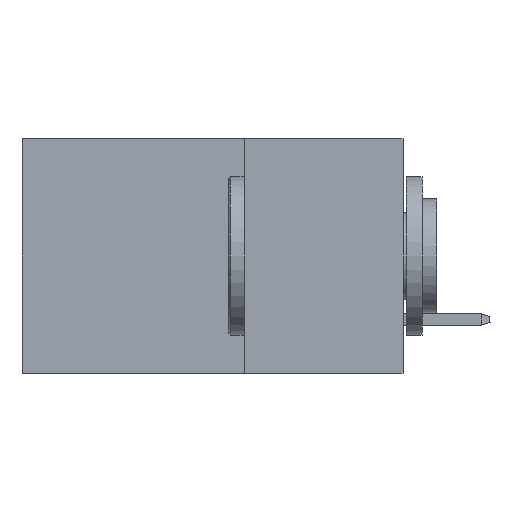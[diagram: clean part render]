
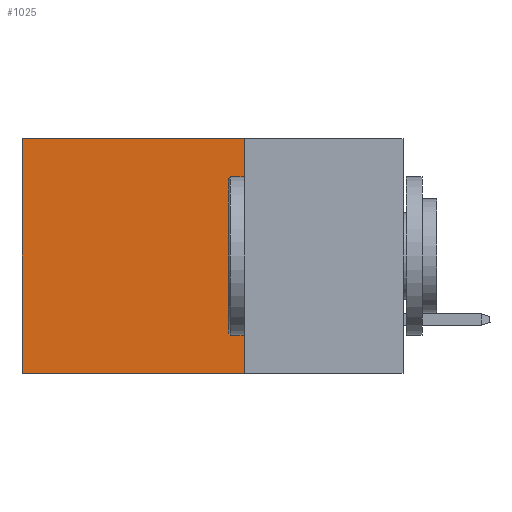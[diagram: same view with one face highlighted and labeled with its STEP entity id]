
A CAD part, left-side view. The second image highlights one B-rep face of the part: STEP entity #1025.
In plain terms, the highlighted planar face has unit normal (-1, 0, 0).
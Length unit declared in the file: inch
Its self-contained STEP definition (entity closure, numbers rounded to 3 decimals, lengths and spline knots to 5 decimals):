
#1025 = ADVANCED_FACE ( 'NONE', ( #2403 ), #2308, .F. ) ;
#1068 = VERTEX_POINT ( 'NONE', #7116 ) ;
#2308 = PLANE ( 'NONE',  #19722 ) ;
#2403 = FACE_OUTER_BOUND ( 'NONE', #3462, .T. ) ;
#2892 = DIRECTION ( 'NONE',  ( 0., 0., -1. ) ) ;
#2958 = CARTESIAN_POINT ( 'NONE',  ( 0.2875, 0.6, 0. ) ) ;
#3462 = EDGE_LOOP ( 'NONE', ( #7460, #17928, #17292, #18241 ) ) ;
#3877 = VERTEX_POINT ( 'NONE', #2958 ) ;
#3930 = VECTOR ( 'NONE', #2892, 39.37008 ) ;
#3978 = CARTESIAN_POINT ( 'NONE',  ( 0.2875, 0.25, 0. ) ) ;
#4448 = LINE ( 'NONE', #9032, #3930 ) ;
#4828 = DIRECTION ( 'NONE',  ( 0., 1., 0. ) ) ;
#5218 = DIRECTION ( 'NONE',  ( 0., 1., 0. ) ) ;
#5452 = CARTESIAN_POINT ( 'NONE',  ( 0.2875, 0.6, -0.37 ) ) ;
#7116 = CARTESIAN_POINT ( 'NONE',  ( 0.2875, 0.25, 0. ) ) ;
#7460 = ORIENTED_EDGE ( 'NONE', *, *, #8730, .T. ) ;
#8002 = VECTOR ( 'NONE', #4828, 39.37008 ) ;
#8730 = EDGE_CURVE ( 'NONE', #3877, #17366, #10065, .T. ) ;
#8749 = VERTEX_POINT ( 'NONE', #11554 ) ;
#9032 = CARTESIAN_POINT ( 'NONE',  ( 0.2875, 0.25, 0. ) ) ;
#9423 = EDGE_CURVE ( 'NONE', #1068, #3877, #19507, .T. ) ;
#9871 = DIRECTION ( 'NONE',  ( 0., 0., -1. ) ) ;
#10065 = LINE ( 'NONE', #10273, #12408 ) ;
#10273 = CARTESIAN_POINT ( 'NONE',  ( 0.2875, 0.6, 0. ) ) ;
#11129 = VECTOR ( 'NONE', #5218, 39.37008 ) ;
#11554 = CARTESIAN_POINT ( 'NONE',  ( 0.2875, 0.25, -0.37 ) ) ;
#12408 = VECTOR ( 'NONE', #9871, 39.37008 ) ;
#12731 = LINE ( 'NONE', #19136, #8002 ) ;
#15348 = EDGE_CURVE ( 'NONE', #1068, #8749, #4448, .T. ) ;
#15640 = CARTESIAN_POINT ( 'NONE',  ( 0.2875, 0.25, 0. ) ) ;
#16382 = DIRECTION ( 'NONE',  ( 1., 0., 0. ) ) ;
#17292 = ORIENTED_EDGE ( 'NONE', *, *, #15348, .F. ) ;
#17366 = VERTEX_POINT ( 'NONE', #5452 ) ;
#17928 = ORIENTED_EDGE ( 'NONE', *, *, #19811, .F. ) ;
#18241 = ORIENTED_EDGE ( 'NONE', *, *, #9423, .T. ) ;
#19136 = CARTESIAN_POINT ( 'NONE',  ( 0.2875, 0.25, -0.37 ) ) ;
#19507 = LINE ( 'NONE', #15640, #11129 ) ;
#19722 = AXIS2_PLACEMENT_3D ( 'NONE', #3978, #16382, #19832 ) ;
#19811 = EDGE_CURVE ( 'NONE', #8749, #17366, #12731, .T. ) ;
#19832 = DIRECTION ( 'NONE',  ( 0., 0., -1. ) ) ;
